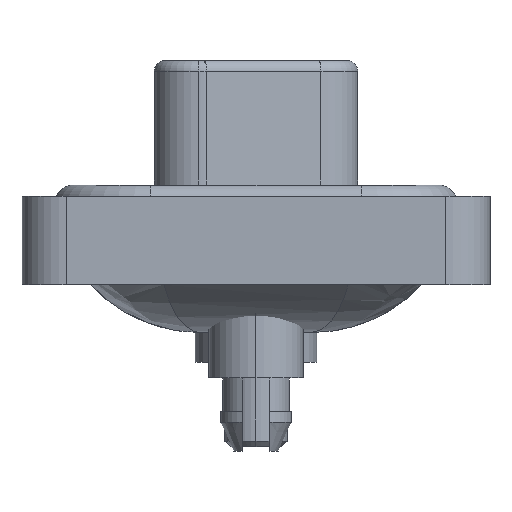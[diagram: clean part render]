
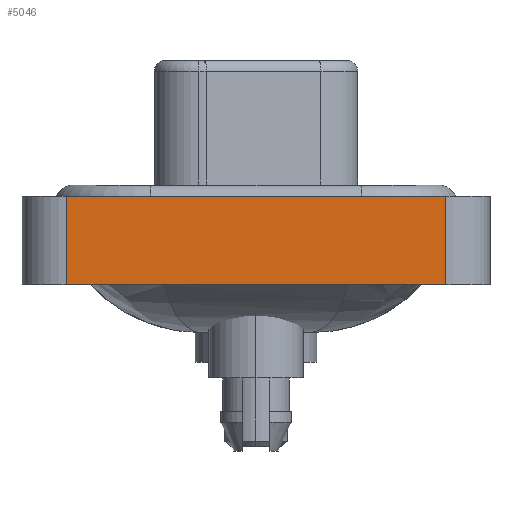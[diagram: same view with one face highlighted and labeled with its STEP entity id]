
A CAD part, left-side view. The second image highlights one B-rep face of the part: STEP entity #5046.
In plain terms, the highlighted planar face has unit normal (-1, 0, 0).
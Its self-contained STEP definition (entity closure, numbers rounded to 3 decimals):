
#67 = VECTOR ( 'NONE', #17970, 1000. ) ;
#106 = CARTESIAN_POINT ( 'NONE',  ( -7.35, 8.55, 0.4 ) ) ;
#3602 = EDGE_LOOP ( 'NONE', ( #7872, #18283, #8685, #12305 ) ) ;
#4597 = CARTESIAN_POINT ( 'NONE',  ( -7.35, -8.55, 0.4 ) ) ;
#4803 = DIRECTION ( 'NONE',  ( 0., 0., 1. ) ) ;
#4987 = PLANE ( 'NONE',  #18093 ) ;
#5046 = ADVANCED_FACE ( 'NONE', ( #10534 ), #4987, .T. ) ;
#5879 = CARTESIAN_POINT ( 'NONE',  ( -7.35, -8.55, -3.6 ) ) ;
#5890 = EDGE_CURVE ( 'NONE', #14290, #12370, #12242, .T. ) ;
#7031 = CARTESIAN_POINT ( 'NONE',  ( -7.35, -8.55, 0.4 ) ) ;
#7215 = LINE ( 'NONE', #11781, #16981 ) ;
#7220 = LINE ( 'NONE', #7031, #17384 ) ;
#7470 = DIRECTION ( 'NONE',  ( 0., 0., 1. ) ) ;
#7679 = CARTESIAN_POINT ( 'NONE',  ( -7.35, -8.55, -3.6 ) ) ;
#7872 = ORIENTED_EDGE ( 'NONE', *, *, #5890, .T. ) ;
#8685 = ORIENTED_EDGE ( 'NONE', *, *, #17998, .F. ) ;
#9587 = LINE ( 'NONE', #12446, #67 ) ;
#10534 = FACE_OUTER_BOUND ( 'NONE', #3602, .T. ) ;
#11781 = CARTESIAN_POINT ( 'NONE',  ( -7.35, -8.55, -3.6 ) ) ;
#12242 = LINE ( 'NONE', #7679, #13719 ) ;
#12305 = ORIENTED_EDGE ( 'NONE', *, *, #15207, .T. ) ;
#12370 = VERTEX_POINT ( 'NONE', #4597 ) ;
#12446 = CARTESIAN_POINT ( 'NONE',  ( -7.35, 8.55, -3.6 ) ) ;
#13054 = DIRECTION ( 'NONE',  ( 0., -1., 0. ) ) ;
#13224 = VERTEX_POINT ( 'NONE', #14246 ) ;
#13679 = CARTESIAN_POINT ( 'NONE',  ( -7.35, -8.55, -3.6 ) ) ;
#13719 = VECTOR ( 'NONE', #4803, 1000. ) ;
#14246 = CARTESIAN_POINT ( 'NONE',  ( -7.35, 8.55, -3.6 ) ) ;
#14290 = VERTEX_POINT ( 'NONE', #5879 ) ;
#14306 = VERTEX_POINT ( 'NONE', #106 ) ;
#15207 = EDGE_CURVE ( 'NONE', #13224, #14290, #7215, .T. ) ;
#16616 = DIRECTION ( 'NONE',  ( -1., 0., 0. ) ) ;
#16981 = VECTOR ( 'NONE', #17606, 1000. ) ;
#17384 = VECTOR ( 'NONE', #13054, 1000. ) ;
#17606 = DIRECTION ( 'NONE',  ( 0., -1., 0. ) ) ;
#17776 = EDGE_CURVE ( 'NONE', #14306, #12370, #7220, .T. ) ;
#17970 = DIRECTION ( 'NONE',  ( 0., 0., 1. ) ) ;
#17998 = EDGE_CURVE ( 'NONE', #13224, #14306, #9587, .T. ) ;
#18093 = AXIS2_PLACEMENT_3D ( 'NONE', #13679, #16616, #7470 ) ;
#18283 = ORIENTED_EDGE ( 'NONE', *, *, #17776, .F. ) ;
